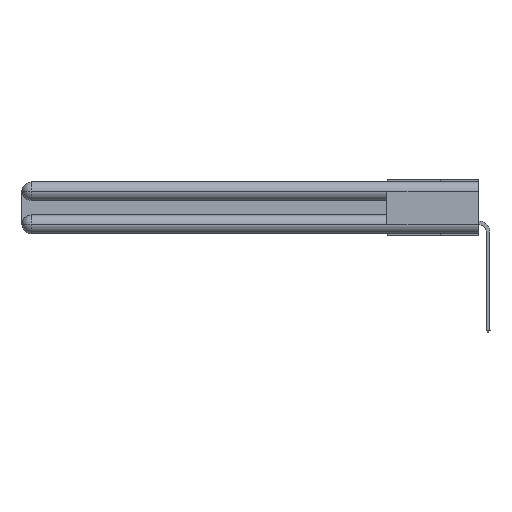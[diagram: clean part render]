
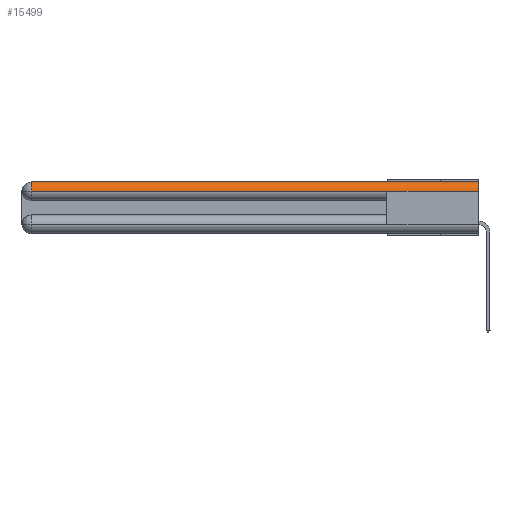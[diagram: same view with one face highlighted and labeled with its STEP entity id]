
A CAD part, left-side view. The second image highlights one B-rep face of the part: STEP entity #15499.
In plain terms, the highlighted cylindrical face has radius 1.562 mm (diameter 3.124 mm), a partial arc.
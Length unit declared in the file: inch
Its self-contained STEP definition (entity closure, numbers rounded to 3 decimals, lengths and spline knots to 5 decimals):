
#299 = LINE ( 'NONE', #9318, #7528 ) ;
#793 = EDGE_CURVE ( 'NONE', #24938, #27607, #13958, .T. ) ;
#1348 = CARTESIAN_POINT ( 'NONE',  ( 0.0615, 2.94, 0. ) ) ;
#1797 = CARTESIAN_POINT ( 'NONE',  ( 0., 0., -0.0615 ) ) ;
#2015 = CARTESIAN_POINT ( 'NONE',  ( 0.0615, 2.94, -0.0615 ) ) ;
#2862 = VERTEX_POINT ( 'NONE', #28647 ) ;
#3453 = CARTESIAN_POINT ( 'NONE',  ( 0., 2.94, -0.0615 ) ) ;
#3702 = DIRECTION ( 'NONE',  ( 1., 0., 0. ) ) ;
#3959 = DIRECTION ( 'NONE',  ( 0., -1., 0. ) ) ;
#4191 = VERTEX_POINT ( 'NONE', #1348 ) ;
#5077 = CARTESIAN_POINT ( 'NONE',  ( 0.0615, 0., -0.0615 ) ) ;
#6059 = AXIS2_PLACEMENT_3D ( 'NONE', #2015, #14965, #25318 ) ;
#7528 = VECTOR ( 'NONE', #11892, 39.37008 ) ;
#8187 = DIRECTION ( 'NONE',  ( 0., 1., 0. ) ) ;
#9318 = CARTESIAN_POINT ( 'NONE',  ( 0.0615, 0., 0. ) ) ;
#9466 = VECTOR ( 'NONE', #8187, 39.37008 ) ;
#10544 = CYLINDRICAL_SURFACE ( 'NONE', #15863, 0.0615 ) ;
#11374 = CARTESIAN_POINT ( 'NONE',  ( 0., 3., -0.0615 ) ) ;
#11892 = DIRECTION ( 'NONE',  ( 0., -1., 0. ) ) ;
#13958 = LINE ( 'NONE', #11374, #29291 ) ;
#13972 = ORIENTED_EDGE ( 'NONE', *, *, #33260, .T. ) ;
#14965 = DIRECTION ( 'NONE',  ( 0., -1., 0. ) ) ;
#15114 = ORIENTED_EDGE ( 'NONE', *, *, #793, .T. ) ;
#15499 = ADVANCED_FACE ( 'NONE', ( #33093 ), #10544, .T. ) ;
#15640 = CIRCLE ( 'NONE', #15990, 0.0615 ) ;
#15863 = AXIS2_PLACEMENT_3D ( 'NONE', #5077, #30735, #32964 ) ;
#15990 = AXIS2_PLACEMENT_3D ( 'NONE', #24400, #16529, #3702 ) ;
#16081 = CARTESIAN_POINT ( 'NONE',  ( 0., 3., -0.0615 ) ) ;
#16529 = DIRECTION ( 'NONE',  ( 0., -1., 0. ) ) ;
#17113 = ORIENTED_EDGE ( 'NONE', *, *, #28343, .F. ) ;
#20263 = EDGE_LOOP ( 'NONE', ( #22839, #13972, #15114, #17113, #24882 ) ) ;
#21297 = CIRCLE ( 'NONE', #6059, 0.0615 ) ;
#21950 = LINE ( 'NONE', #16081, #9466 ) ;
#22839 = ORIENTED_EDGE ( 'NONE', *, *, #27544, .F. ) ;
#24400 = CARTESIAN_POINT ( 'NONE',  ( 0.0615, 0., -0.0615 ) ) ;
#24530 = VERTEX_POINT ( 'NONE', #1797 ) ;
#24882 = ORIENTED_EDGE ( 'NONE', *, *, #33218, .F. ) ;
#24938 = VERTEX_POINT ( 'NONE', #3453 ) ;
#25042 = CARTESIAN_POINT ( 'NONE',  ( 0., 0.6, -0.0615 ) ) ;
#25318 = DIRECTION ( 'NONE',  ( 0., 0., 1. ) ) ;
#27544 = EDGE_CURVE ( 'NONE', #4191, #2862, #299, .T. ) ;
#27607 = VERTEX_POINT ( 'NONE', #25042 ) ;
#28343 = EDGE_CURVE ( 'NONE', #24530, #27607, #21950, .T. ) ;
#28647 = CARTESIAN_POINT ( 'NONE',  ( 0.0615, 0., 0. ) ) ;
#29291 = VECTOR ( 'NONE', #3959, 39.37008 ) ;
#30735 = DIRECTION ( 'NONE',  ( 0., 1., 0. ) ) ;
#32964 = DIRECTION ( 'NONE',  ( 0., 0., 1. ) ) ;
#33093 = FACE_OUTER_BOUND ( 'NONE', #20263, .T. ) ;
#33218 = EDGE_CURVE ( 'NONE', #2862, #24530, #15640, .T. ) ;
#33260 = EDGE_CURVE ( 'NONE', #4191, #24938, #21297, .T. ) ;
